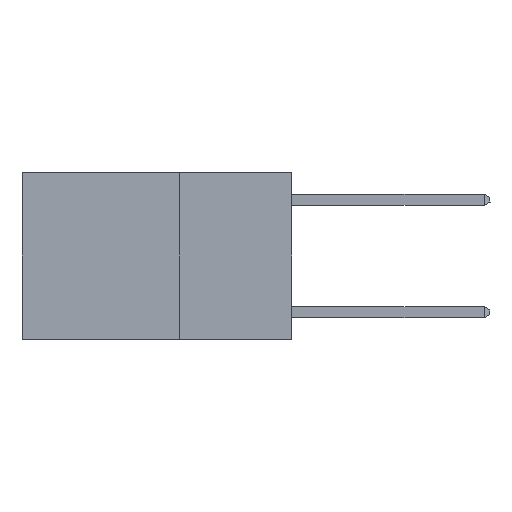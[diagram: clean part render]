
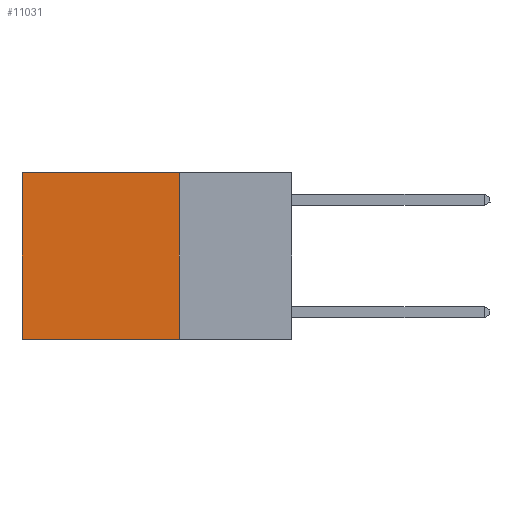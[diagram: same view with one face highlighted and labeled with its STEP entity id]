
A CAD part, left-side view. The second image highlights one B-rep face of the part: STEP entity #11031.
In plain terms, the highlighted planar face has unit normal (-1, 0, 0).
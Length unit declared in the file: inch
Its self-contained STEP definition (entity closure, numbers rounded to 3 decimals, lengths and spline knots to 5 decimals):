
#36 = AXIS2_PLACEMENT_3D ( 'NONE', #3113, #11444, #4297 ) ;
#383 = VERTEX_POINT ( 'NONE', #11924 ) ;
#1123 = LINE ( 'NONE', #2457, #3660 ) ;
#1228 = VERTEX_POINT ( 'NONE', #5529 ) ;
#1295 = CARTESIAN_POINT ( 'NONE',  ( 0.2625, 0.25, 0. ) ) ;
#2203 = VERTEX_POINT ( 'NONE', #4153 ) ;
#2457 = CARTESIAN_POINT ( 'NONE',  ( 0.2625, 0.25, 0. ) ) ;
#2514 = EDGE_CURVE ( 'NONE', #383, #2203, #1123, .T. ) ;
#2575 = DIRECTION ( 'NONE',  ( 0., 1., 0. ) ) ;
#3113 = CARTESIAN_POINT ( 'NONE',  ( 0.2625, 0.25, 0. ) ) ;
#3528 = DIRECTION ( 'NONE',  ( 0., 1., 0. ) ) ;
#3539 = FACE_OUTER_BOUND ( 'NONE', #15278, .T. ) ;
#3660 = VECTOR ( 'NONE', #4865, 39.37008 ) ;
#3776 = DIRECTION ( 'NONE',  ( 0., 0., -1. ) ) ;
#4153 = CARTESIAN_POINT ( 'NONE',  ( 0.2625, 0.25, -0.37 ) ) ;
#4297 = DIRECTION ( 'NONE',  ( 0., 0., -1. ) ) ;
#4865 = DIRECTION ( 'NONE',  ( 0., 0., -1. ) ) ;
#5013 = LINE ( 'NONE', #10707, #11026 ) ;
#5529 = CARTESIAN_POINT ( 'NONE',  ( 0.2625, 0.6, 0. ) ) ;
#5617 = ORIENTED_EDGE ( 'NONE', *, *, #6824, .T. ) ;
#6345 = VECTOR ( 'NONE', #2575, 39.37008 ) ;
#6681 = EDGE_CURVE ( 'NONE', #2203, #11901, #5013, .T. ) ;
#6773 = ORIENTED_EDGE ( 'NONE', *, *, #6681, .F. ) ;
#6824 = EDGE_CURVE ( 'NONE', #1228, #11901, #11923, .T. ) ;
#7158 = ORIENTED_EDGE ( 'NONE', *, *, #9861, .T. ) ;
#7855 = PLANE ( 'NONE',  #36 ) ;
#8765 = VECTOR ( 'NONE', #3776, 39.37008 ) ;
#9758 = CARTESIAN_POINT ( 'NONE',  ( 0.2625, 0.6, 0. ) ) ;
#9861 = EDGE_CURVE ( 'NONE', #383, #1228, #9927, .T. ) ;
#9927 = LINE ( 'NONE', #1295, #6345 ) ;
#10707 = CARTESIAN_POINT ( 'NONE',  ( 0.2625, 0.25, -0.37 ) ) ;
#11026 = VECTOR ( 'NONE', #3528, 39.37008 ) ;
#11031 = ADVANCED_FACE ( 'NONE', ( #3539 ), #7855, .F. ) ;
#11444 = DIRECTION ( 'NONE',  ( 1., 0., 0. ) ) ;
#11901 = VERTEX_POINT ( 'NONE', #15207 ) ;
#11923 = LINE ( 'NONE', #9758, #8765 ) ;
#11924 = CARTESIAN_POINT ( 'NONE',  ( 0.2625, 0.25, 0. ) ) ;
#13069 = ORIENTED_EDGE ( 'NONE', *, *, #2514, .F. ) ;
#15207 = CARTESIAN_POINT ( 'NONE',  ( 0.2625, 0.6, -0.37 ) ) ;
#15278 = EDGE_LOOP ( 'NONE', ( #5617, #6773, #13069, #7158 ) ) ;
